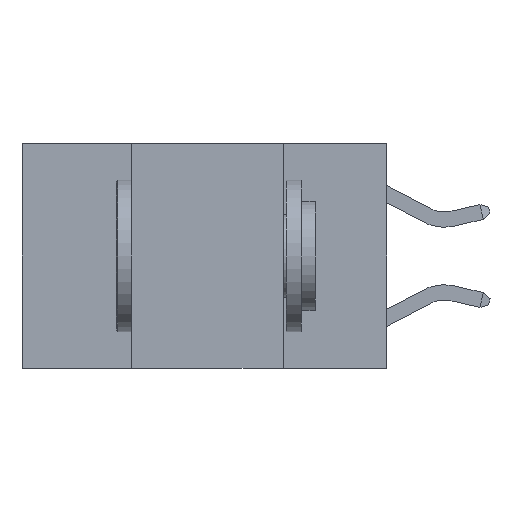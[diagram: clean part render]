
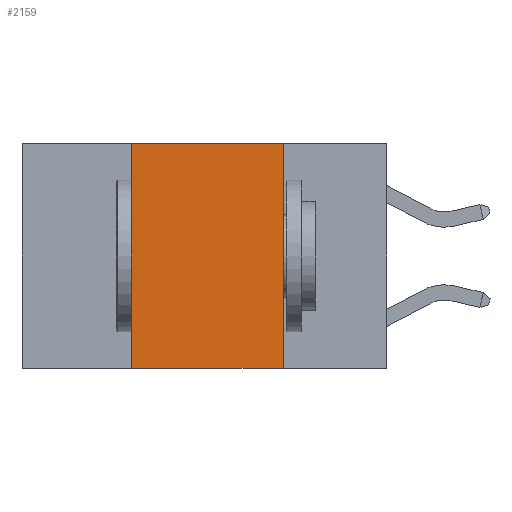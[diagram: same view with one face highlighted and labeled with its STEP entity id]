
A CAD part, left-side view. The second image highlights one B-rep face of the part: STEP entity #2159.
In plain terms, the highlighted planar face has unit normal (-1, 0, 0).
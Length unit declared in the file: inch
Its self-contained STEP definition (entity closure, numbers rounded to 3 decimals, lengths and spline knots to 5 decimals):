
#58 = VECTOR ( 'NONE', #4446, 39.37008 ) ;
#438 = DIRECTION ( 'NONE',  ( 0., 0., -1. ) ) ;
#588 = CARTESIAN_POINT ( 'NONE',  ( 0., 0.42, 0. ) ) ;
#808 = VECTOR ( 'NONE', #2145, 39.37008 ) ;
#931 = EDGE_CURVE ( 'NONE', #4288, #5716, #9087, .T. ) ;
#1561 = CARTESIAN_POINT ( 'NONE',  ( 0., 0.6, 0. ) ) ;
#1700 = VECTOR ( 'NONE', #5221, 39.37008 ) ;
#1845 = EDGE_CURVE ( 'NONE', #6382, #1897, #4594, .T. ) ;
#1897 = VERTEX_POINT ( 'NONE', #8161 ) ;
#2145 = DIRECTION ( 'NONE',  ( 0., 0., 1. ) ) ;
#2159 = ADVANCED_FACE ( 'NONE', ( #2282 ), #5664, .F. ) ;
#2193 = CARTESIAN_POINT ( 'NONE',  ( 0., 0.6, -0.37 ) ) ;
#2276 = CARTESIAN_POINT ( 'NONE',  ( 0., 0.17, 0. ) ) ;
#2282 = FACE_OUTER_BOUND ( 'NONE', #2296, .T. ) ;
#2296 = EDGE_LOOP ( 'NONE', ( #7387, #7505, #7673, #8381 ) ) ;
#2321 = DIRECTION ( 'NONE',  ( 0., -1., 0. ) ) ;
#2745 = EDGE_CURVE ( 'NONE', #6382, #5716, #4809, .T. ) ;
#3340 = VECTOR ( 'NONE', #2321, 39.37008 ) ;
#4288 = VERTEX_POINT ( 'NONE', #2276 ) ;
#4446 = DIRECTION ( 'NONE',  ( 0., -1., 0. ) ) ;
#4594 = LINE ( 'NONE', #588, #808 ) ;
#4809 = LINE ( 'NONE', #2193, #58 ) ;
#4956 = DIRECTION ( 'NONE',  ( 1., 0., 0. ) ) ;
#5221 = DIRECTION ( 'NONE',  ( 0., 0., -1. ) ) ;
#5242 = CARTESIAN_POINT ( 'NONE',  ( 0., 0.17, 0. ) ) ;
#5664 = PLANE ( 'NONE',  #5769 ) ;
#5716 = VERTEX_POINT ( 'NONE', #6785 ) ;
#5769 = AXIS2_PLACEMENT_3D ( 'NONE', #7132, #4956, #438 ) ;
#6382 = VERTEX_POINT ( 'NONE', #8180 ) ;
#6785 = CARTESIAN_POINT ( 'NONE',  ( 0., 0.17, -0.37 ) ) ;
#7132 = CARTESIAN_POINT ( 'NONE',  ( 0., 0.6, 0. ) ) ;
#7387 = ORIENTED_EDGE ( 'NONE', *, *, #931, .F. ) ;
#7505 = ORIENTED_EDGE ( 'NONE', *, *, #9273, .F. ) ;
#7673 = ORIENTED_EDGE ( 'NONE', *, *, #1845, .F. ) ;
#8161 = CARTESIAN_POINT ( 'NONE',  ( 0., 0.42, 0. ) ) ;
#8180 = CARTESIAN_POINT ( 'NONE',  ( 0., 0.42, -0.37 ) ) ;
#8381 = ORIENTED_EDGE ( 'NONE', *, *, #2745, .T. ) ;
#9087 = LINE ( 'NONE', #5242, #1700 ) ;
#9211 = LINE ( 'NONE', #1561, #3340 ) ;
#9273 = EDGE_CURVE ( 'NONE', #1897, #4288, #9211, .T. ) ;
